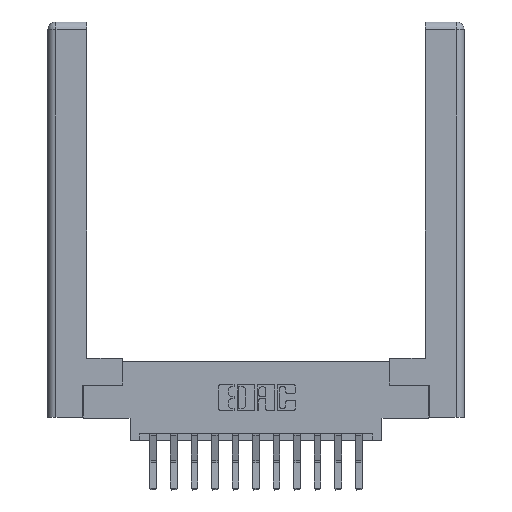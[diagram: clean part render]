
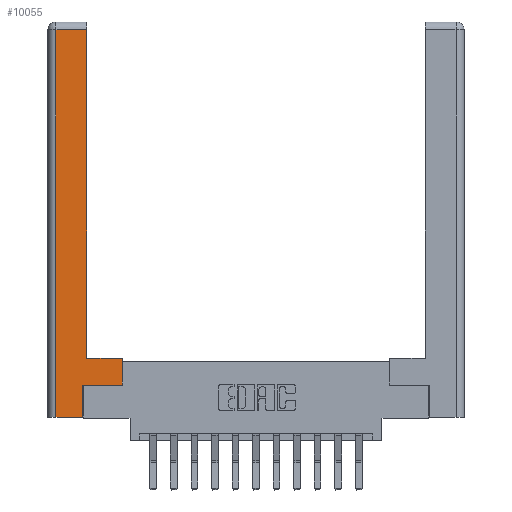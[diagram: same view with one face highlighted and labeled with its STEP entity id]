
A CAD part, top view. The second image highlights one B-rep face of the part: STEP entity #10055.
In plain terms, the highlighted planar face has unit normal (0, 0, 1).
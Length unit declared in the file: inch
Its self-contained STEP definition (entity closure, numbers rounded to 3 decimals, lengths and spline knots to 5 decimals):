
#28 = VECTOR ( 'NONE', #5912, 39.37008 ) ;
#449 = ORIENTED_EDGE ( 'NONE', *, *, #5539, .T. ) ;
#985 = LINE ( 'NONE', #4950, #2853 ) ;
#1368 = VERTEX_POINT ( 'NONE', #10048 ) ;
#1467 = ORIENTED_EDGE ( 'NONE', *, *, #14594, .T. ) ;
#1625 = ORIENTED_EDGE ( 'NONE', *, *, #12424, .T. ) ;
#1627 = LINE ( 'NONE', #6910, #10408 ) ;
#2164 = CARTESIAN_POINT ( 'NONE',  ( 0.265, 0.245, 0. ) ) ;
#2251 = LINE ( 'NONE', #6966, #28 ) ;
#2402 = LINE ( 'NONE', #13595, #6715 ) ;
#2417 = CARTESIAN_POINT ( 'NONE',  ( 0.265, 0., 0. ) ) ;
#2677 = EDGE_LOOP ( 'NONE', ( #3269, #6814, #12195, #449, #11505, #1467, #1625, #2726 ) ) ;
#2726 = ORIENTED_EDGE ( 'NONE', *, *, #13168, .T. ) ;
#2783 = AXIS2_PLACEMENT_3D ( 'NONE', #15045, #7952, #15093 ) ;
#2853 = VECTOR ( 'NONE', #7582, 39.37008 ) ;
#3269 = ORIENTED_EDGE ( 'NONE', *, *, #5730, .T. ) ;
#4950 = CARTESIAN_POINT ( 'NONE',  ( 0.0615, 0., 0. ) ) ;
#5159 = VERTEX_POINT ( 'NONE', #2164 ) ;
#5347 = CARTESIAN_POINT ( 'NONE',  ( 0.0615, 0., 0. ) ) ;
#5539 = EDGE_CURVE ( 'NONE', #15170, #7845, #8908, .T. ) ;
#5700 = VECTOR ( 'NONE', #13853, 39.37008 ) ;
#5730 = EDGE_CURVE ( 'NONE', #14646, #10430, #1627, .T. ) ;
#5779 = VERTEX_POINT ( 'NONE', #5905 ) ;
#5905 = CARTESIAN_POINT ( 'NONE',  ( 0.565, 0.245, 0. ) ) ;
#5912 = DIRECTION ( 'NONE',  ( -1., 0., 0. ) ) ;
#6007 = CARTESIAN_POINT ( 'NONE',  ( 0.565, 0.45, 0. ) ) ;
#6403 = DIRECTION ( 'NONE',  ( 0., 1., 0. ) ) ;
#6466 = LINE ( 'NONE', #7664, #8150 ) ;
#6715 = VECTOR ( 'NONE', #6403, 39.37008 ) ;
#6814 = ORIENTED_EDGE ( 'NONE', *, *, #9603, .T. ) ;
#6910 = CARTESIAN_POINT ( 'NONE',  ( 0.295, 3., 0. ) ) ;
#6966 = CARTESIAN_POINT ( 'NONE',  ( 0.295, 0.45, 0. ) ) ;
#7151 = DIRECTION ( 'NONE',  ( 1., 0., 0. ) ) ;
#7582 = DIRECTION ( 'NONE',  ( 0., -1., 0. ) ) ;
#7664 = CARTESIAN_POINT ( 'NONE',  ( 0.0615, 2.94, 0. ) ) ;
#7762 = FACE_OUTER_BOUND ( 'NONE', #2677, .T. ) ;
#7845 = VERTEX_POINT ( 'NONE', #2417 ) ;
#7952 = DIRECTION ( 'NONE',  ( 0., 0., -1. ) ) ;
#8145 = CARTESIAN_POINT ( 'NONE',  ( 0.265, 0., 0. ) ) ;
#8150 = VECTOR ( 'NONE', #12465, 39.37008 ) ;
#8619 = CARTESIAN_POINT ( 'NONE',  ( 0.565, 0.45, 0. ) ) ;
#8824 = LINE ( 'NONE', #6007, #11613 ) ;
#8908 = LINE ( 'NONE', #8145, #5700 ) ;
#9567 = VERTEX_POINT ( 'NONE', #8619 ) ;
#9603 = EDGE_CURVE ( 'NONE', #10430, #1368, #6466, .T. ) ;
#10048 = CARTESIAN_POINT ( 'NONE',  ( 0.0615, 2.94, 0. ) ) ;
#10055 = ADVANCED_FACE ( 'NONE', ( #7762 ), #13871, .F. ) ;
#10408 = VECTOR ( 'NONE', #12052, 39.37008 ) ;
#10430 = VERTEX_POINT ( 'NONE', #12209 ) ;
#10792 = EDGE_CURVE ( 'NONE', #1368, #15170, #985, .T. ) ;
#10844 = DIRECTION ( 'NONE',  ( 0., 1., 0. ) ) ;
#11505 = ORIENTED_EDGE ( 'NONE', *, *, #14435, .T. ) ;
#11613 = VECTOR ( 'NONE', #10844, 39.37008 ) ;
#11863 = CARTESIAN_POINT ( 'NONE',  ( 0.565, 0.245, 0. ) ) ;
#12052 = DIRECTION ( 'NONE',  ( 0., 1., 0. ) ) ;
#12195 = ORIENTED_EDGE ( 'NONE', *, *, #10792, .T. ) ;
#12209 = CARTESIAN_POINT ( 'NONE',  ( 0.295, 2.94, 0. ) ) ;
#12424 = EDGE_CURVE ( 'NONE', #5779, #9567, #8824, .T. ) ;
#12465 = DIRECTION ( 'NONE',  ( -1., 0., 0. ) ) ;
#13168 = EDGE_CURVE ( 'NONE', #9567, #14646, #2251, .T. ) ;
#13595 = CARTESIAN_POINT ( 'NONE',  ( 0.265, 0.245, 0. ) ) ;
#13853 = DIRECTION ( 'NONE',  ( 1., 0., 0. ) ) ;
#13871 = PLANE ( 'NONE',  #2783 ) ;
#14346 = VECTOR ( 'NONE', #7151, 39.37008 ) ;
#14377 = CARTESIAN_POINT ( 'NONE',  ( 0.295, 0.45, 0. ) ) ;
#14435 = EDGE_CURVE ( 'NONE', #7845, #5159, #2402, .T. ) ;
#14594 = EDGE_CURVE ( 'NONE', #5159, #5779, #15064, .T. ) ;
#14646 = VERTEX_POINT ( 'NONE', #14377 ) ;
#15045 = CARTESIAN_POINT ( 'NONE',  ( 0., 0., 0. ) ) ;
#15064 = LINE ( 'NONE', #11863, #14346 ) ;
#15093 = DIRECTION ( 'NONE',  ( -1., 0., 0. ) ) ;
#15170 = VERTEX_POINT ( 'NONE', #5347 ) ;
